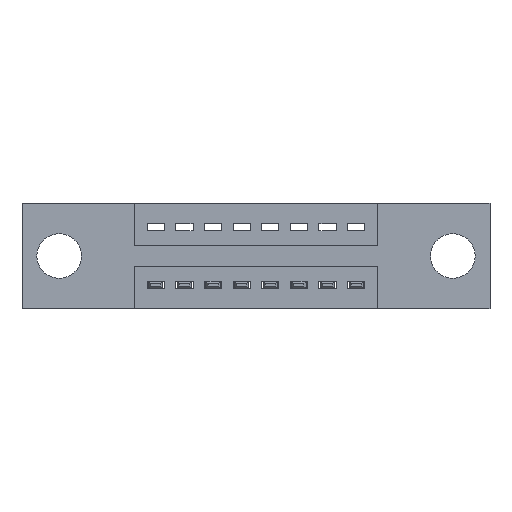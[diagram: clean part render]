
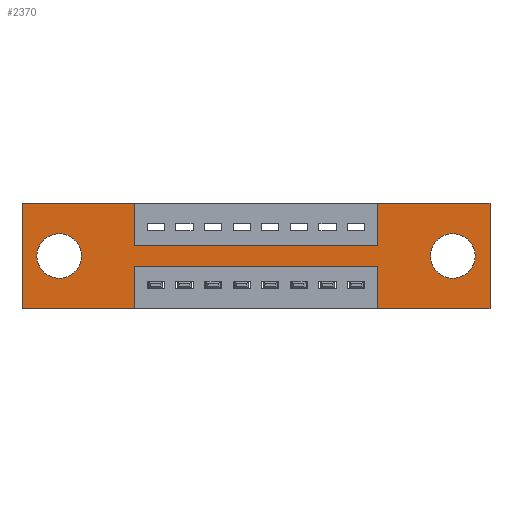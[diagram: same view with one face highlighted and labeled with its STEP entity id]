
A CAD part, front view. The second image highlights one B-rep face of the part: STEP entity #2370.
In plain terms, the highlighted planar face has unit normal (0, -1, 0).
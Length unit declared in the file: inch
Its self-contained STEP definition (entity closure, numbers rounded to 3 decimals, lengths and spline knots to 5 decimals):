
#63 = ORIENTED_EDGE ( 'NONE', *, *, #6191, .F. ) ;
#160 = CARTESIAN_POINT ( 'NONE',  ( 1.505, 0., -0.185 ) ) ;
#173 = CIRCLE ( 'NONE', #6193, 0.078 ) ;
#192 = DIRECTION ( 'NONE',  ( 0., 1., 0. ) ) ;
#271 = ORIENTED_EDGE ( 'NONE', *, *, #3128, .T. ) ;
#280 = EDGE_CURVE ( 'NONE', #3140, #3927, #8896, .T. ) ;
#284 = CARTESIAN_POINT ( 'NONE',  ( 0., 0., 0. ) ) ;
#379 = CARTESIAN_POINT ( 'NONE',  ( 1.505, 0., -0.107 ) ) ;
#458 = EDGE_CURVE ( 'NONE', #6963, #1763, #8000, .T. ) ;
#545 = DIRECTION ( 'NONE',  ( 0., 0., 1. ) ) ;
#567 = CARTESIAN_POINT ( 'NONE',  ( 0.3925, 0., -0.15 ) ) ;
#592 = ORIENTED_EDGE ( 'NONE', *, *, #9199, .T. ) ;
#620 = CARTESIAN_POINT ( 'NONE',  ( 0., 0., 0. ) ) ;
#1016 = VECTOR ( 'NONE', #10123, 39.37008 ) ;
#1223 = VERTEX_POINT ( 'NONE', #284 ) ;
#1312 = CARTESIAN_POINT ( 'NONE',  ( 0.13, 0., -0.185 ) ) ;
#1360 = DIRECTION ( 'NONE',  ( -1., 0., 0. ) ) ;
#1438 = CARTESIAN_POINT ( 'NONE',  ( 1.505, 0., -0.263 ) ) ;
#1457 = CARTESIAN_POINT ( 'NONE',  ( 0., 0., -0.37 ) ) ;
#1624 = ORIENTED_EDGE ( 'NONE', *, *, #5924, .F. ) ;
#1763 = VERTEX_POINT ( 'NONE', #7021 ) ;
#1837 = DIRECTION ( 'NONE',  ( 0., 1., 0. ) ) ;
#1965 = LINE ( 'NONE', #3625, #9963 ) ;
#2024 = CARTESIAN_POINT ( 'NONE',  ( 0.3925, 0., 0. ) ) ;
#2118 = CARTESIAN_POINT ( 'NONE',  ( 1.635, 0., 0. ) ) ;
#2165 = CARTESIAN_POINT ( 'NONE',  ( 0.13, 0., -0.263 ) ) ;
#2261 = DIRECTION ( 'NONE',  ( 0., 0., 1. ) ) ;
#2370 = ADVANCED_FACE ( 'NONE', ( #5142, #2954, #6910 ), #6673, .T. ) ;
#2440 = VERTEX_POINT ( 'NONE', #2571 ) ;
#2451 = CARTESIAN_POINT ( 'NONE',  ( 0., 0., 0. ) ) ;
#2464 = DIRECTION ( 'NONE',  ( 1., 0., 0. ) ) ;
#2571 = CARTESIAN_POINT ( 'NONE',  ( 1.635, 0., -0.37 ) ) ;
#2608 = CARTESIAN_POINT ( 'NONE',  ( 1.2425, 0., 0. ) ) ;
#2643 = CARTESIAN_POINT ( 'NONE',  ( 0.3925, 0., -0.22 ) ) ;
#2647 = DIRECTION ( 'NONE',  ( 0., 1., 0. ) ) ;
#2894 = ORIENTED_EDGE ( 'NONE', *, *, #5630, .F. ) ;
#2954 = FACE_BOUND ( 'NONE', #6409, .T. ) ;
#3016 = EDGE_LOOP ( 'NONE', ( #6304, #4479, #8154, #1624, #2894, #9035, #4842, #6859, #8593, #63, #4578, #6620 ) ) ;
#3074 = ORIENTED_EDGE ( 'NONE', *, *, #8408, .T. ) ;
#3128 = EDGE_CURVE ( 'NONE', #8837, #3438, #6452, .T. ) ;
#3140 = VERTEX_POINT ( 'NONE', #4643 ) ;
#3194 = CARTESIAN_POINT ( 'NONE',  ( 1.2425, 0., -0.37 ) ) ;
#3203 = LINE ( 'NONE', #1457, #9061 ) ;
#3400 = DIRECTION ( 'NONE',  ( 0., 0., -1. ) ) ;
#3433 = VERTEX_POINT ( 'NONE', #2643 ) ;
#3438 = VERTEX_POINT ( 'NONE', #379 ) ;
#3444 = DIRECTION ( 'NONE',  ( 0., 0., -1. ) ) ;
#3494 = LINE ( 'NONE', #6654, #9324 ) ;
#3577 = VECTOR ( 'NONE', #4475, 39.37008 ) ;
#3606 = LINE ( 'NONE', #8088, #9642 ) ;
#3625 = CARTESIAN_POINT ( 'NONE',  ( 0., 0., -0.37 ) ) ;
#3692 = DIRECTION ( 'NONE',  ( -1., 0., 0. ) ) ;
#3767 = EDGE_CURVE ( 'NONE', #3927, #6963, #10406, .T. ) ;
#3823 = LINE ( 'NONE', #620, #7691 ) ;
#3878 = VERTEX_POINT ( 'NONE', #2118 ) ;
#3892 = DIRECTION ( 'NONE',  ( 1., 0., 0. ) ) ;
#3927 = VERTEX_POINT ( 'NONE', #567 ) ;
#3939 = CARTESIAN_POINT ( 'NONE',  ( 0.3925, 0., -0.15 ) ) ;
#3988 = VECTOR ( 'NONE', #7963, 39.37008 ) ;
#4102 = DIRECTION ( 'NONE',  ( 0., 0., 1. ) ) ;
#4218 = VECTOR ( 'NONE', #2464, 39.37008 ) ;
#4427 = CARTESIAN_POINT ( 'NONE',  ( 0.13, 0., -0.107 ) ) ;
#4464 = CARTESIAN_POINT ( 'NONE',  ( 1.635, 0., 0. ) ) ;
#4475 = DIRECTION ( 'NONE',  ( 0., 0., -1. ) ) ;
#4479 = ORIENTED_EDGE ( 'NONE', *, *, #7746, .F. ) ;
#4538 = VERTEX_POINT ( 'NONE', #9585 ) ;
#4578 = ORIENTED_EDGE ( 'NONE', *, *, #6447, .F. ) ;
#4643 = CARTESIAN_POINT ( 'NONE',  ( 0.3925, 0., 0. ) ) ;
#4842 = ORIENTED_EDGE ( 'NONE', *, *, #458, .F. ) ;
#4939 = VECTOR ( 'NONE', #3400, 39.37008 ) ;
#4967 = EDGE_CURVE ( 'NONE', #1763, #3878, #9754, .T. ) ;
#5142 = FACE_BOUND ( 'NONE', #8695, .T. ) ;
#5630 = EDGE_CURVE ( 'NONE', #3878, #2440, #7711, .T. ) ;
#5777 = CARTESIAN_POINT ( 'NONE',  ( 0.3925, 0., -0.22 ) ) ;
#5782 = VECTOR ( 'NONE', #4102, 39.37008 ) ;
#5800 = EDGE_CURVE ( 'NONE', #8345, #8753, #1965, .T. ) ;
#5924 = EDGE_CURVE ( 'NONE', #2440, #6559, #3203, .T. ) ;
#6191 = EDGE_CURVE ( 'NONE', #1223, #3140, #8727, .T. ) ;
#6193 = AXIS2_PLACEMENT_3D ( 'NONE', #1312, #7045, #2261 ) ;
#6249 = CIRCLE ( 'NONE', #8849, 0.078 ) ;
#6298 = VERTEX_POINT ( 'NONE', #2165 ) ;
#6304 = ORIENTED_EDGE ( 'NONE', *, *, #10220, .F. ) ;
#6374 = CARTESIAN_POINT ( 'NONE',  ( 0., 0., -0.37 ) ) ;
#6409 = EDGE_LOOP ( 'NONE', ( #3074, #8284 ) ) ;
#6447 = EDGE_CURVE ( 'NONE', #8753, #1223, #3823, .T. ) ;
#6452 = CIRCLE ( 'NONE', #9277, 0.078 ) ;
#6559 = VERTEX_POINT ( 'NONE', #3194 ) ;
#6620 = ORIENTED_EDGE ( 'NONE', *, *, #5800, .F. ) ;
#6654 = CARTESIAN_POINT ( 'NONE',  ( 1.2425, 0., -0.37 ) ) ;
#6673 = PLANE ( 'NONE',  #10121 ) ;
#6699 = CARTESIAN_POINT ( 'NONE',  ( 1.505, 0., -0.185 ) ) ;
#6779 = VECTOR ( 'NONE', #3892, 39.37008 ) ;
#6859 = ORIENTED_EDGE ( 'NONE', *, *, #3767, .F. ) ;
#6910 = FACE_OUTER_BOUND ( 'NONE', #3016, .T. ) ;
#6963 = VERTEX_POINT ( 'NONE', #7645 ) ;
#7021 = CARTESIAN_POINT ( 'NONE',  ( 1.2425, 0., 0. ) ) ;
#7045 = DIRECTION ( 'NONE',  ( 0., 1., 0. ) ) ;
#7046 = CARTESIAN_POINT ( 'NONE',  ( 0., 0., -0.37 ) ) ;
#7320 = LINE ( 'NONE', #5777, #1016 ) ;
#7383 = CARTESIAN_POINT ( 'NONE',  ( 0.13, 0., -0.185 ) ) ;
#7431 = AXIS2_PLACEMENT_3D ( 'NONE', #7383, #2647, #8147 ) ;
#7453 = DIRECTION ( 'NONE',  ( 0., 0., -1. ) ) ;
#7645 = CARTESIAN_POINT ( 'NONE',  ( 1.2425, 0., -0.15 ) ) ;
#7691 = VECTOR ( 'NONE', #545, 39.37008 ) ;
#7711 = LINE ( 'NONE', #4464, #3577 ) ;
#7746 = EDGE_CURVE ( 'NONE', #4538, #3433, #7320, .T. ) ;
#7963 = DIRECTION ( 'NONE',  ( 1., 0., 0. ) ) ;
#7988 = DIRECTION ( 'NONE',  ( 0., 0., -1. ) ) ;
#8000 = LINE ( 'NONE', #2608, #5782 ) ;
#8016 = CARTESIAN_POINT ( 'NONE',  ( 0.3925, 0., -0.37 ) ) ;
#8088 = CARTESIAN_POINT ( 'NONE',  ( 0.3925, 0., -0.37 ) ) ;
#8147 = DIRECTION ( 'NONE',  ( 0., 0., 1. ) ) ;
#8154 = ORIENTED_EDGE ( 'NONE', *, *, #9807, .F. ) ;
#8284 = ORIENTED_EDGE ( 'NONE', *, *, #9504, .T. ) ;
#8345 = VERTEX_POINT ( 'NONE', #8016 ) ;
#8408 = EDGE_CURVE ( 'NONE', #9068, #6298, #8697, .T. ) ;
#8593 = ORIENTED_EDGE ( 'NONE', *, *, #280, .F. ) ;
#8695 = EDGE_LOOP ( 'NONE', ( #592, #271 ) ) ;
#8697 = CIRCLE ( 'NONE', #7431, 0.078 ) ;
#8727 = LINE ( 'NONE', #2451, #4218 ) ;
#8753 = VERTEX_POINT ( 'NONE', #7046 ) ;
#8837 = VERTEX_POINT ( 'NONE', #1438 ) ;
#8849 = AXIS2_PLACEMENT_3D ( 'NONE', #6699, #1837, #7453 ) ;
#8896 = LINE ( 'NONE', #2024, #4939 ) ;
#8912 = CARTESIAN_POINT ( 'NONE',  ( 0., 0., 0. ) ) ;
#8935 = DIRECTION ( 'NONE',  ( 0., -1., 0. ) ) ;
#9035 = ORIENTED_EDGE ( 'NONE', *, *, #4967, .F. ) ;
#9061 = VECTOR ( 'NONE', #1360, 39.37008 ) ;
#9068 = VERTEX_POINT ( 'NONE', #4427 ) ;
#9199 = EDGE_CURVE ( 'NONE', #3438, #8837, #6249, .T. ) ;
#9277 = AXIS2_PLACEMENT_3D ( 'NONE', #160, #192, #9878 ) ;
#9324 = VECTOR ( 'NONE', #9589, 39.37008 ) ;
#9504 = EDGE_CURVE ( 'NONE', #6298, #9068, #173, .T. ) ;
#9585 = CARTESIAN_POINT ( 'NONE',  ( 1.2425, 0., -0.22 ) ) ;
#9589 = DIRECTION ( 'NONE',  ( 0., 0., 1. ) ) ;
#9642 = VECTOR ( 'NONE', #3444, 39.37008 ) ;
#9754 = LINE ( 'NONE', #8912, #3988 ) ;
#9807 = EDGE_CURVE ( 'NONE', #6559, #4538, #3494, .T. ) ;
#9878 = DIRECTION ( 'NONE',  ( 0., 0., -1. ) ) ;
#9963 = VECTOR ( 'NONE', #3692, 39.37008 ) ;
#10121 = AXIS2_PLACEMENT_3D ( 'NONE', #6374, #8935, #7988 ) ;
#10123 = DIRECTION ( 'NONE',  ( -1., 0., 0. ) ) ;
#10220 = EDGE_CURVE ( 'NONE', #3433, #8345, #3606, .T. ) ;
#10406 = LINE ( 'NONE', #3939, #6779 ) ;
